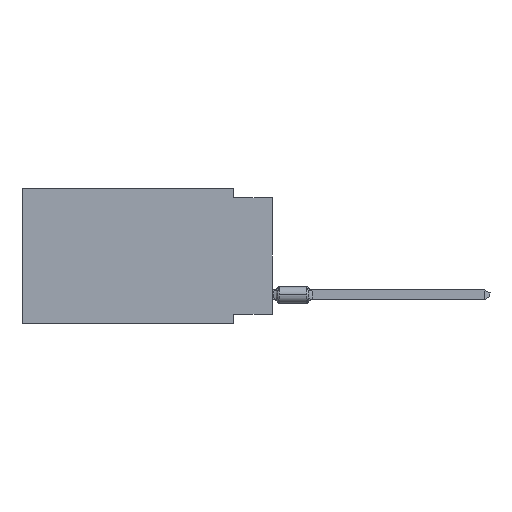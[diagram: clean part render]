
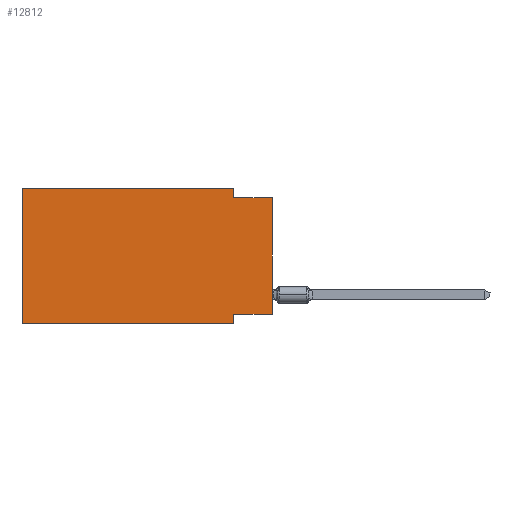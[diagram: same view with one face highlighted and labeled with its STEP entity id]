
A CAD part, left-side view. The second image highlights one B-rep face of the part: STEP entity #12812.
In plain terms, the highlighted planar face has unit normal (-1, 0, 0).
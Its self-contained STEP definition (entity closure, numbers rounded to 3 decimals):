
#2328 = LINE ( 'NONE', #36054, #42448 ) ;
#2526 = ORIENTED_EDGE ( 'NONE', *, *, #46520, .F. ) ;
#4576 = CARTESIAN_POINT ( 'NONE',  ( 0., 16.383, 0. ) ) ;
#4715 = VERTEX_POINT ( 'NONE', #4759 ) ;
#4759 = CARTESIAN_POINT ( 'NONE',  ( 0., 2.54, -0.635 ) ) ;
#6057 = EDGE_CURVE ( 'NONE', #8291, #49031, #39388, .T. ) ;
#7652 = VECTOR ( 'NONE', #47807, 1000. ) ;
#8225 = ORIENTED_EDGE ( 'NONE', *, *, #9507, .F. ) ;
#8291 = VERTEX_POINT ( 'NONE', #45211 ) ;
#9507 = EDGE_CURVE ( 'NONE', #26790, #39305, #12290, .T. ) ;
#9747 = LINE ( 'NONE', #43471, #33372 ) ;
#11177 = VECTOR ( 'NONE', #38609, 1000. ) ;
#11810 = VECTOR ( 'NONE', #41880, 1000. ) ;
#12290 = LINE ( 'NONE', #38296, #11810 ) ;
#12812 = ADVANCED_FACE ( 'NONE', ( #54141 ), #46186, .F. ) ;
#15792 = DIRECTION ( 'NONE',  ( 0., 0., 1. ) ) ;
#17877 = CARTESIAN_POINT ( 'NONE',  ( 0., 0., -0.635 ) ) ;
#19943 = LINE ( 'NONE', #53650, #39887 ) ;
#20877 = EDGE_CURVE ( 'NONE', #49031, #48059, #19943, .T. ) ;
#20971 = CARTESIAN_POINT ( 'NONE',  ( 0., 16.383, 0. ) ) ;
#21875 = LINE ( 'NONE', #27081, #11177 ) ;
#22372 = DIRECTION ( 'NONE',  ( 0., 0., -1. ) ) ;
#22611 = DIRECTION ( 'NONE',  ( 0., 0., 1. ) ) ;
#23194 = CARTESIAN_POINT ( 'NONE',  ( 0., 0., -8.255 ) ) ;
#23587 = EDGE_CURVE ( 'NONE', #25699, #48059, #21875, .T. ) ;
#24820 = DIRECTION ( 'NONE',  ( 1., 0., 0. ) ) ;
#25699 = VERTEX_POINT ( 'NONE', #36778 ) ;
#26790 = VERTEX_POINT ( 'NONE', #4576 ) ;
#26929 = ORIENTED_EDGE ( 'NONE', *, *, #50130, .F. ) ;
#27081 = CARTESIAN_POINT ( 'NONE',  ( 0., 16.383, -8.89 ) ) ;
#27913 = ORIENTED_EDGE ( 'NONE', *, *, #20877, .F. ) ;
#28988 = DIRECTION ( 'NONE',  ( 0., 0., -1. ) ) ;
#30545 = LINE ( 'NONE', #43157, #7652 ) ;
#32827 = CARTESIAN_POINT ( 'NONE',  ( 0., 2.54, 0. ) ) ;
#32828 = VERTEX_POINT ( 'NONE', #17877 ) ;
#33011 = CARTESIAN_POINT ( 'NONE',  ( 0., 2.54, -8.89 ) ) ;
#33108 = AXIS2_PLACEMENT_3D ( 'NONE', #20971, #24820, #41540 ) ;
#33372 = VECTOR ( 'NONE', #22372, 1000. ) ;
#33444 = VECTOR ( 'NONE', #39915, 1000. ) ;
#34139 = EDGE_LOOP ( 'NONE', ( #52403, #2526, #26929, #8225, #41704, #43463, #27913, #36594 ) ) ;
#36054 = CARTESIAN_POINT ( 'NONE',  ( 0., 16.383, 0. ) ) ;
#36594 = ORIENTED_EDGE ( 'NONE', *, *, #6057, .F. ) ;
#36778 = CARTESIAN_POINT ( 'NONE',  ( 0., 16.383, -8.89 ) ) ;
#38296 = CARTESIAN_POINT ( 'NONE',  ( 0., 16.383, 0. ) ) ;
#38609 = DIRECTION ( 'NONE',  ( 0., -1., 0. ) ) ;
#39305 = VERTEX_POINT ( 'NONE', #32827 ) ;
#39388 = LINE ( 'NONE', #23194, #33444 ) ;
#39887 = VECTOR ( 'NONE', #28988, 1000. ) ;
#39915 = DIRECTION ( 'NONE',  ( 0., 1., 0. ) ) ;
#41540 = DIRECTION ( 'NONE',  ( 0., 0., -1. ) ) ;
#41704 = ORIENTED_EDGE ( 'NONE', *, *, #43462, .F. ) ;
#41880 = DIRECTION ( 'NONE',  ( 0., -1., 0. ) ) ;
#42380 = EDGE_CURVE ( 'NONE', #8291, #32828, #49770, .T. ) ;
#42448 = VECTOR ( 'NONE', #22611, 1000. ) ;
#43157 = CARTESIAN_POINT ( 'NONE',  ( 0., 0., -0.635 ) ) ;
#43462 = EDGE_CURVE ( 'NONE', #25699, #26790, #2328, .T. ) ;
#43463 = ORIENTED_EDGE ( 'NONE', *, *, #23587, .T. ) ;
#43471 = CARTESIAN_POINT ( 'NONE',  ( 0., 2.54, 0. ) ) ;
#43730 = CARTESIAN_POINT ( 'NONE',  ( 0., 2.54, -8.255 ) ) ;
#45211 = CARTESIAN_POINT ( 'NONE',  ( 0., 0., -8.255 ) ) ;
#45803 = VECTOR ( 'NONE', #15792, 1000. ) ;
#46186 = PLANE ( 'NONE',  #33108 ) ;
#46520 = EDGE_CURVE ( 'NONE', #4715, #32828, #30545, .T. ) ;
#47807 = DIRECTION ( 'NONE',  ( 0., -1., 0. ) ) ;
#48059 = VERTEX_POINT ( 'NONE', #33011 ) ;
#49031 = VERTEX_POINT ( 'NONE', #43730 ) ;
#49770 = LINE ( 'NONE', #53339, #45803 ) ;
#50130 = EDGE_CURVE ( 'NONE', #39305, #4715, #9747, .T. ) ;
#52403 = ORIENTED_EDGE ( 'NONE', *, *, #42380, .T. ) ;
#53339 = CARTESIAN_POINT ( 'NONE',  ( 0., 0., 0. ) ) ;
#53650 = CARTESIAN_POINT ( 'NONE',  ( 0., 2.54, -8.89 ) ) ;
#54141 = FACE_OUTER_BOUND ( 'NONE', #34139, .T. ) ;
